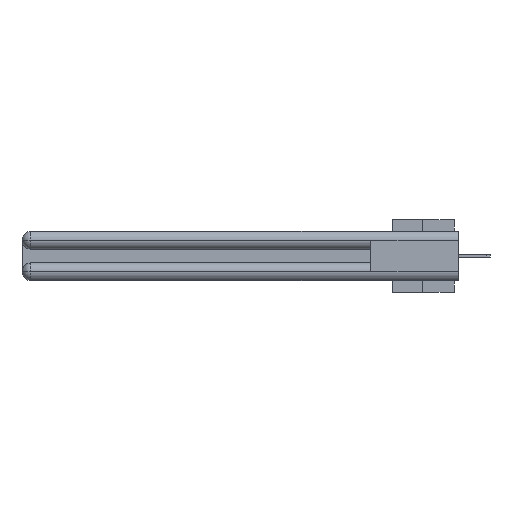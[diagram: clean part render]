
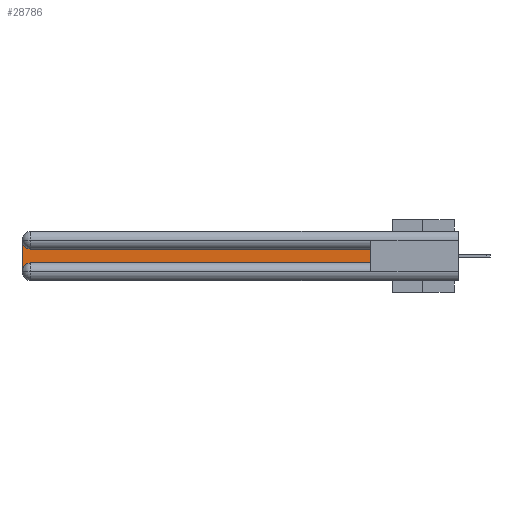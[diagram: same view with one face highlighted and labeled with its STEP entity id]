
A CAD part, left-side view. The second image highlights one B-rep face of the part: STEP entity #28786.
In plain terms, the highlighted planar face has unit normal (-1, 0, 0).
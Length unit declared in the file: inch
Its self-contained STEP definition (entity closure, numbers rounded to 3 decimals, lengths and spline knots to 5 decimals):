
#229 = EDGE_LOOP ( 'NONE', ( #8664, #14312, #13729, #20922, #26679, #20446 ) ) ;
#266 = DIRECTION ( 'NONE',  ( 0., 0., -1. ) ) ;
#989 = CARTESIAN_POINT ( 'NONE',  ( 0.075, 3., -0.1225 ) ) ;
#1048 = EDGE_CURVE ( 'NONE', #27389, #7885, #3985, .T. ) ;
#1702 = DIRECTION ( 'NONE',  ( 0., 0., 1. ) ) ;
#2758 = VERTEX_POINT ( 'NONE', #3518 ) ;
#2885 = AXIS2_PLACEMENT_3D ( 'NONE', #989, #8481, #25175 ) ;
#3357 = LINE ( 'NONE', #29237, #21886 ) ;
#3518 = CARTESIAN_POINT ( 'NONE',  ( 0.075, 0.6, -0.1225 ) ) ;
#3985 = CIRCLE ( 'NONE', #24041, 0.06 ) ;
#5485 = EDGE_CURVE ( 'NONE', #28274, #22483, #8395, .T. ) ;
#5571 = LINE ( 'NONE', #6439, #25503 ) ;
#5926 = VERTEX_POINT ( 'NONE', #23692 ) ;
#6439 = CARTESIAN_POINT ( 'NONE',  ( 0.075, 0.6, -0.2175 ) ) ;
#7885 = VERTEX_POINT ( 'NONE', #24422 ) ;
#7907 = CARTESIAN_POINT ( 'NONE',  ( 0.075, 2.94, -0.1225 ) ) ;
#8365 = PLANE ( 'NONE',  #2885 ) ;
#8395 = CIRCLE ( 'NONE', #10337, 0.06 ) ;
#8462 = EDGE_CURVE ( 'NONE', #2758, #27389, #16323, .T. ) ;
#8481 = DIRECTION ( 'NONE',  ( 1., 0., 0. ) ) ;
#8664 = ORIENTED_EDGE ( 'NONE', *, *, #8462, .T. ) ;
#8977 = DIRECTION ( 'NONE',  ( 0., -1., 0. ) ) ;
#9201 = VECTOR ( 'NONE', #31324, 39.37008 ) ;
#10337 = AXIS2_PLACEMENT_3D ( 'NONE', #12337, #28987, #14716 ) ;
#12337 = CARTESIAN_POINT ( 'NONE',  ( 0.075, 2.94, -0.2775 ) ) ;
#12744 = EDGE_CURVE ( 'NONE', #22483, #5926, #5571, .T. ) ;
#13729 = ORIENTED_EDGE ( 'NONE', *, *, #29750, .T. ) ;
#14312 = ORIENTED_EDGE ( 'NONE', *, *, #1048, .T. ) ;
#14716 = DIRECTION ( 'NONE',  ( 0., 0., -1. ) ) ;
#15028 = DIRECTION ( 'NONE',  ( 1., 0., 0. ) ) ;
#16323 = LINE ( 'NONE', #17007, #9201 ) ;
#17007 = CARTESIAN_POINT ( 'NONE',  ( 0.075, 0.6, -0.1225 ) ) ;
#17196 = LINE ( 'NONE', #18669, #23518 ) ;
#18669 = CARTESIAN_POINT ( 'NONE',  ( 0.075, 0.6, -0.2175 ) ) ;
#19325 = FACE_OUTER_BOUND ( 'NONE', #229, .T. ) ;
#20446 = ORIENTED_EDGE ( 'NONE', *, *, #26886, .T. ) ;
#20922 = ORIENTED_EDGE ( 'NONE', *, *, #5485, .T. ) ;
#21886 = VECTOR ( 'NONE', #266, 39.37008 ) ;
#22483 = VERTEX_POINT ( 'NONE', #30552 ) ;
#23518 = VECTOR ( 'NONE', #1702, 39.37008 ) ;
#23692 = CARTESIAN_POINT ( 'NONE',  ( 0.075, 0.6, -0.2175 ) ) ;
#24041 = AXIS2_PLACEMENT_3D ( 'NONE', #27157, #15028, #24809 ) ;
#24422 = CARTESIAN_POINT ( 'NONE',  ( 0.075, 3., -0.0625 ) ) ;
#24809 = DIRECTION ( 'NONE',  ( 0., 0., -1. ) ) ;
#25175 = DIRECTION ( 'NONE',  ( 0., 0., -1. ) ) ;
#25503 = VECTOR ( 'NONE', #8977, 39.37008 ) ;
#25635 = CARTESIAN_POINT ( 'NONE',  ( 0.075, 3., -0.2775 ) ) ;
#26679 = ORIENTED_EDGE ( 'NONE', *, *, #12744, .T. ) ;
#26886 = EDGE_CURVE ( 'NONE', #5926, #2758, #17196, .T. ) ;
#27157 = CARTESIAN_POINT ( 'NONE',  ( 0.075, 2.94, -0.0625 ) ) ;
#27389 = VERTEX_POINT ( 'NONE', #7907 ) ;
#28274 = VERTEX_POINT ( 'NONE', #25635 ) ;
#28786 = ADVANCED_FACE ( 'NONE', ( #19325 ), #8365, .F. ) ;
#28987 = DIRECTION ( 'NONE',  ( 1., 0., 0. ) ) ;
#29237 = CARTESIAN_POINT ( 'NONE',  ( 0.075, 3., -0.2175 ) ) ;
#29750 = EDGE_CURVE ( 'NONE', #7885, #28274, #3357, .T. ) ;
#30552 = CARTESIAN_POINT ( 'NONE',  ( 0.075, 2.94, -0.2175 ) ) ;
#31324 = DIRECTION ( 'NONE',  ( 0., 1., 0. ) ) ;
